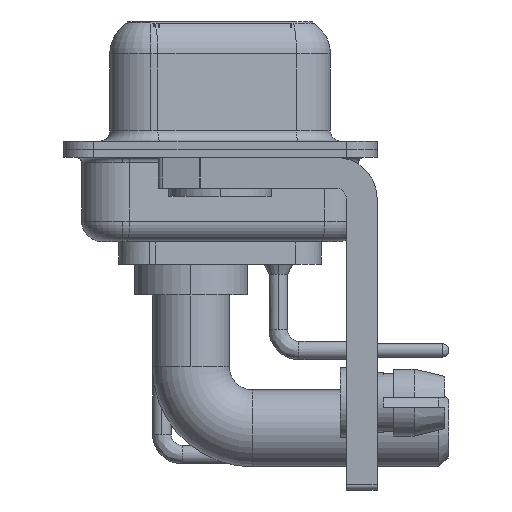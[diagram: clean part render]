
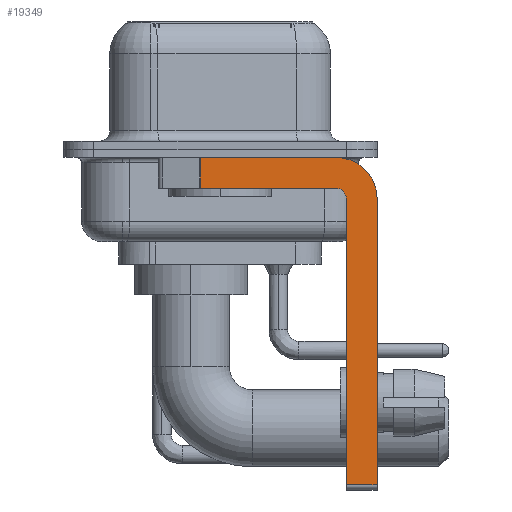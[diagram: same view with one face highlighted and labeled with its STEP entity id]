
A CAD part, left-side view. The second image highlights one B-rep face of the part: STEP entity #19349.
In plain terms, the highlighted planar face has unit normal (-1, 0, 0).
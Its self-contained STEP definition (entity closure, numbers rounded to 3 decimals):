
#244 = EDGE_CURVE ( 'NONE', #6712, #19113, #24248, .T. ) ;
#258 = CARTESIAN_POINT ( 'NONE',  ( -2.9, -7.65, -2.4 ) ) ;
#853 = CARTESIAN_POINT ( 'NONE',  ( -2.9, -5.65, -2.4 ) ) ;
#1721 = EDGE_CURVE ( 'NONE', #24397, #23583, #17520, .T. ) ;
#1730 = CARTESIAN_POINT ( 'NONE',  ( -2.9, -5.65, -1.9 ) ) ;
#1890 = LINE ( 'NONE', #6700, #11653 ) ;
#2180 = ORIENTED_EDGE ( 'NONE', *, *, #3156, .F. ) ;
#3017 = CARTESIAN_POINT ( 'NONE',  ( -2.9, -5.65, -1.9 ) ) ;
#3156 = EDGE_CURVE ( 'NONE', #31510, #8206, #27293, .T. ) ;
#3207 = CARTESIAN_POINT ( 'NONE',  ( -2.9, 0.978, -0.4 ) ) ;
#3401 = FACE_OUTER_BOUND ( 'NONE', #27928, .T. ) ;
#3530 = DIRECTION ( 'NONE',  ( 0., -1., 0. ) ) ;
#3618 = VERTEX_POINT ( 'NONE', #15654 ) ;
#3931 = ORIENTED_EDGE ( 'NONE', *, *, #1721, .F. ) ;
#4739 = DIRECTION ( 'NONE',  ( 0., -1., 0. ) ) ;
#5300 = DIRECTION ( 'NONE',  ( 0., 0., 1. ) ) ;
#5426 = DIRECTION ( 'NONE',  ( 1., 0., 0. ) ) ;
#6633 = CARTESIAN_POINT ( 'NONE',  ( -2.9, 0.978, -1.9 ) ) ;
#6700 = CARTESIAN_POINT ( 'NONE',  ( -2.9, -7.65, -2.4 ) ) ;
#6712 = VERTEX_POINT ( 'NONE', #3207 ) ;
#6743 = AXIS2_PLACEMENT_3D ( 'NONE', #25954, #15700, #8450 ) ;
#8206 = VERTEX_POINT ( 'NONE', #24067 ) ;
#8450 = DIRECTION ( 'NONE',  ( 0., 0., 1. ) ) ;
#9503 = ORIENTED_EDGE ( 'NONE', *, *, #16607, .F. ) ;
#10257 = CARTESIAN_POINT ( 'NONE',  ( -2.9, -5.65, -2.4 ) ) ;
#11350 = EDGE_CURVE ( 'NONE', #23583, #3618, #1890, .T. ) ;
#11653 = VECTOR ( 'NONE', #12012, 1000. ) ;
#12012 = DIRECTION ( 'NONE',  ( 0., 0., -1. ) ) ;
#12988 = ORIENTED_EDGE ( 'NONE', *, *, #20712, .F. ) ;
#13160 = EDGE_CURVE ( 'NONE', #6712, #24397, #29766, .T. ) ;
#14852 = VECTOR ( 'NONE', #21361, 1000. ) ;
#15654 = CARTESIAN_POINT ( 'NONE',  ( -2.9, -7.65, -16.35 ) ) ;
#15700 = DIRECTION ( 'NONE',  ( -1., 0., 0. ) ) ;
#16607 = EDGE_CURVE ( 'NONE', #8206, #26359, #18041, .T. ) ;
#16816 = LINE ( 'NONE', #1730, #21846 ) ;
#17323 = VECTOR ( 'NONE', #4739, 1000. ) ;
#17450 = EDGE_CURVE ( 'NONE', #31510, #3618, #23605, .T. ) ;
#17496 = ORIENTED_EDGE ( 'NONE', *, *, #244, .T. ) ;
#17520 = CIRCLE ( 'NONE', #28254, 2. ) ;
#18041 = CIRCLE ( 'NONE', #6743, 0.5 ) ;
#19113 = VERTEX_POINT ( 'NONE', #6633 ) ;
#19349 = ADVANCED_FACE ( 'NONE', ( #3401 ), #25076, .F. ) ;
#20712 = EDGE_CURVE ( 'NONE', #26359, #19113, #16816, .T. ) ;
#21317 = DIRECTION ( 'NONE',  ( 0., 1., 0. ) ) ;
#21361 = DIRECTION ( 'NONE',  ( 0., 0., -1. ) ) ;
#21846 = VECTOR ( 'NONE', #21317, 1000. ) ;
#22803 = AXIS2_PLACEMENT_3D ( 'NONE', #853, #23162, #27809 ) ;
#23162 = DIRECTION ( 'NONE',  ( 1., 0., 0. ) ) ;
#23440 = CARTESIAN_POINT ( 'NONE',  ( -2.9, -5.65, -16.35 ) ) ;
#23583 = VERTEX_POINT ( 'NONE', #258 ) ;
#23605 = LINE ( 'NONE', #23440, #24247 ) ;
#23770 = CARTESIAN_POINT ( 'NONE',  ( -2.9, 0.978, -1.9 ) ) ;
#23837 = ORIENTED_EDGE ( 'NONE', *, *, #13160, .F. ) ;
#24067 = CARTESIAN_POINT ( 'NONE',  ( -2.9, -6.15, -2.4 ) ) ;
#24247 = VECTOR ( 'NONE', #3530, 1000. ) ;
#24248 = LINE ( 'NONE', #23770, #14852 ) ;
#24397 = VERTEX_POINT ( 'NONE', #31162 ) ;
#25028 = CARTESIAN_POINT ( 'NONE',  ( -2.9, -6.15, -16.6 ) ) ;
#25076 = PLANE ( 'NONE',  #22803 ) ;
#25954 = CARTESIAN_POINT ( 'NONE',  ( -2.9, -5.65, -2.4 ) ) ;
#26359 = VERTEX_POINT ( 'NONE', #3017 ) ;
#26733 = CARTESIAN_POINT ( 'NONE',  ( -2.9, 3., -0.4 ) ) ;
#26892 = ORIENTED_EDGE ( 'NONE', *, *, #17450, .T. ) ;
#27293 = LINE ( 'NONE', #25028, #27330 ) ;
#27330 = VECTOR ( 'NONE', #5300, 1000. ) ;
#27364 = CARTESIAN_POINT ( 'NONE',  ( -2.9, -6.15, -16.35 ) ) ;
#27809 = DIRECTION ( 'NONE',  ( 0., 0., -1. ) ) ;
#27928 = EDGE_LOOP ( 'NONE', ( #23837, #17496, #12988, #9503, #2180, #26892, #29729, #3931 ) ) ;
#28254 = AXIS2_PLACEMENT_3D ( 'NONE', #10257, #5426, #29677 ) ;
#29677 = DIRECTION ( 'NONE',  ( 0., 0., -1. ) ) ;
#29729 = ORIENTED_EDGE ( 'NONE', *, *, #11350, .F. ) ;
#29766 = LINE ( 'NONE', #26733, #17323 ) ;
#31162 = CARTESIAN_POINT ( 'NONE',  ( -2.9, -5.65, -0.4 ) ) ;
#31510 = VERTEX_POINT ( 'NONE', #27364 ) ;
